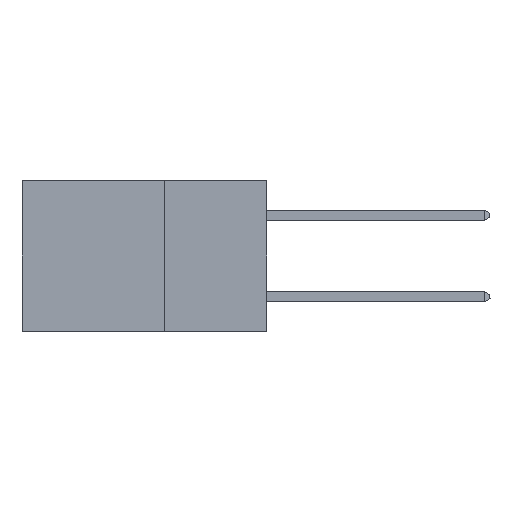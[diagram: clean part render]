
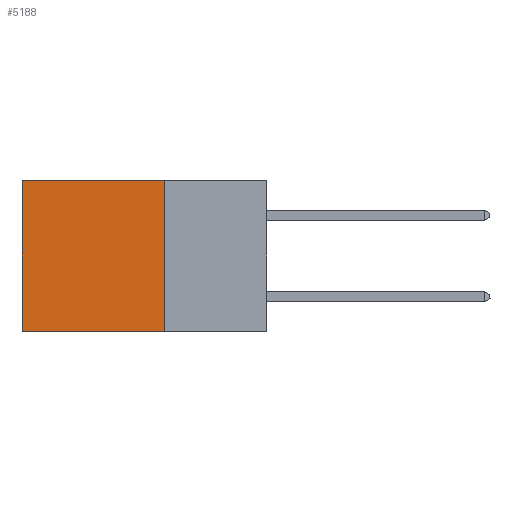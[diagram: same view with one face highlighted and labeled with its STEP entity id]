
A CAD part, left-side view. The second image highlights one B-rep face of the part: STEP entity #5188.
In plain terms, the highlighted planar face has unit normal (-1, 0, 0).
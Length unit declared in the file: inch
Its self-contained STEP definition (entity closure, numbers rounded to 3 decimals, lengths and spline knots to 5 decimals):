
#1302 = LINE ( 'NONE', #9547, #7580 ) ;
#1627 = DIRECTION ( 'NONE',  ( 0., 0., -1. ) ) ;
#1682 = EDGE_CURVE ( 'NONE', #4023, #2703, #13472, .T. ) ;
#1989 = EDGE_LOOP ( 'NONE', ( #2580, #10120, #7825, #2539 ) ) ;
#2308 = DIRECTION ( 'NONE',  ( 0., 1., 0. ) ) ;
#2437 = EDGE_CURVE ( 'NONE', #11295, #11730, #9856, .T. ) ;
#2536 = VECTOR ( 'NONE', #12904, 39.37008 ) ;
#2539 = ORIENTED_EDGE ( 'NONE', *, *, #1682, .T. ) ;
#2580 = ORIENTED_EDGE ( 'NONE', *, *, #10234, .T. ) ;
#2703 = VERTEX_POINT ( 'NONE', #12078 ) ;
#4023 = VERTEX_POINT ( 'NONE', #12237 ) ;
#4944 = VECTOR ( 'NONE', #2308, 39.37008 ) ;
#5188 = ADVANCED_FACE ( 'NONE', ( #12513 ), #8911, .F. ) ;
#6368 = DIRECTION ( 'NONE',  ( 0., 0., -1. ) ) ;
#6644 = CARTESIAN_POINT ( 'NONE',  ( 0.2875, 0.25, 0. ) ) ;
#7580 = VECTOR ( 'NONE', #6368, 39.37008 ) ;
#7714 = CARTESIAN_POINT ( 'NONE',  ( 0.2875, 0.25, 0. ) ) ;
#7825 = ORIENTED_EDGE ( 'NONE', *, *, #13710, .F. ) ;
#7929 = CARTESIAN_POINT ( 'NONE',  ( 0.2875, 0.6, -0.37 ) ) ;
#8911 = PLANE ( 'NONE',  #9281 ) ;
#9259 = CARTESIAN_POINT ( 'NONE',  ( 0.2875, 0.25, -0.37 ) ) ;
#9281 = AXIS2_PLACEMENT_3D ( 'NONE', #6644, #12068, #13270 ) ;
#9368 = LINE ( 'NONE', #10201, #11584 ) ;
#9547 = CARTESIAN_POINT ( 'NONE',  ( 0.2875, 0.6, 0. ) ) ;
#9856 = LINE ( 'NONE', #9259, #2536 ) ;
#10120 = ORIENTED_EDGE ( 'NONE', *, *, #2437, .F. ) ;
#10201 = CARTESIAN_POINT ( 'NONE',  ( 0.2875, 0.25, 0. ) ) ;
#10234 = EDGE_CURVE ( 'NONE', #2703, #11730, #1302, .T. ) ;
#11295 = VERTEX_POINT ( 'NONE', #13747 ) ;
#11584 = VECTOR ( 'NONE', #1627, 39.37008 ) ;
#11730 = VERTEX_POINT ( 'NONE', #7929 ) ;
#12068 = DIRECTION ( 'NONE',  ( 1., 0., 0. ) ) ;
#12078 = CARTESIAN_POINT ( 'NONE',  ( 0.2875, 0.6, 0. ) ) ;
#12237 = CARTESIAN_POINT ( 'NONE',  ( 0.2875, 0.25, 0. ) ) ;
#12513 = FACE_OUTER_BOUND ( 'NONE', #1989, .T. ) ;
#12904 = DIRECTION ( 'NONE',  ( 0., 1., 0. ) ) ;
#13270 = DIRECTION ( 'NONE',  ( 0., 0., -1. ) ) ;
#13472 = LINE ( 'NONE', #7714, #4944 ) ;
#13710 = EDGE_CURVE ( 'NONE', #4023, #11295, #9368, .T. ) ;
#13747 = CARTESIAN_POINT ( 'NONE',  ( 0.2875, 0.25, -0.37 ) ) ;
